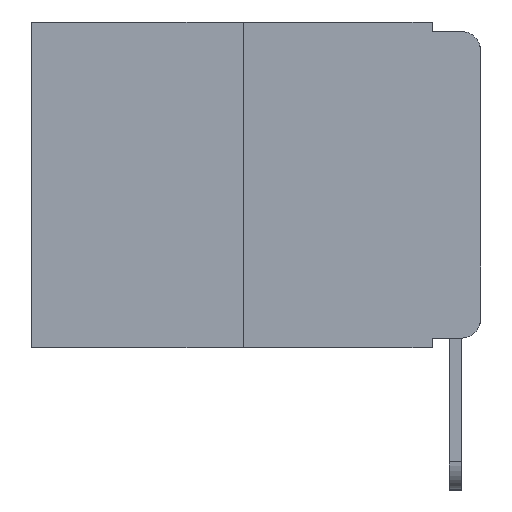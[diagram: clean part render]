
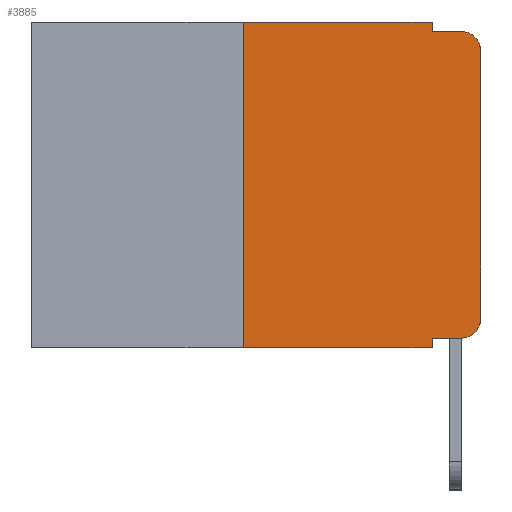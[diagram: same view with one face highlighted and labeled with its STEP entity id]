
A CAD part, left-side view. The second image highlights one B-rep face of the part: STEP entity #3885.
In plain terms, the highlighted planar face has unit normal (-1, 0, 0).
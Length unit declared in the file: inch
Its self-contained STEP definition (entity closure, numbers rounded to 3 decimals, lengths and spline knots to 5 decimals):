
#54 = DIRECTION ( 'NONE',  ( 0., 0., -1. ) ) ;
#356 = EDGE_CURVE ( 'NONE', #2292, #10760, #12862, .T. ) ;
#435 = VERTEX_POINT ( 'NONE', #4787 ) ;
#515 = VECTOR ( 'NONE', #8094, 39.37008 ) ;
#619 = EDGE_CURVE ( 'NONE', #8110, #1332, #3125, .T. ) ;
#902 = CARTESIAN_POINT ( 'NONE',  ( 0., 0.051, 0. ) ) ;
#1042 = ORIENTED_EDGE ( 'NONE', *, *, #1504, .T. ) ;
#1160 = VECTOR ( 'NONE', #5556, 39.37008 ) ;
#1332 = VERTEX_POINT ( 'NONE', #2573 ) ;
#1504 = EDGE_CURVE ( 'NONE', #435, #7835, #13304, .T. ) ;
#1597 = CARTESIAN_POINT ( 'NONE',  ( 0., 0.051, -0.333 ) ) ;
#1759 = EDGE_CURVE ( 'NONE', #7755, #8168, #12975, .T. ) ;
#1916 = PLANE ( 'NONE',  #10055 ) ;
#2100 = EDGE_CURVE ( 'NONE', #435, #2292, #2464, .T. ) ;
#2230 = CARTESIAN_POINT ( 'NONE',  ( 0., 0., -0.03 ) ) ;
#2292 = VERTEX_POINT ( 'NONE', #11133 ) ;
#2399 = CARTESIAN_POINT ( 'NONE',  ( 0., 0.051, -0.343 ) ) ;
#2464 = LINE ( 'NONE', #9834, #5792 ) ;
#2573 = CARTESIAN_POINT ( 'NONE',  ( 0., 0.02, -0.01 ) ) ;
#2598 = DIRECTION ( 'NONE',  ( 0., 0., 1. ) ) ;
#2879 = EDGE_CURVE ( 'NONE', #10760, #8481, #5236, .T. ) ;
#2931 = LINE ( 'NONE', #7078, #10517 ) ;
#3125 = CIRCLE ( 'NONE', #4054, 0.02 ) ;
#3409 = VECTOR ( 'NONE', #5769, 39.37008 ) ;
#3885 = ADVANCED_FACE ( 'NONE', ( #4985 ), #1916, .F. ) ;
#3945 = CARTESIAN_POINT ( 'NONE',  ( 0., 0.473, -0.343 ) ) ;
#4054 = AXIS2_PLACEMENT_3D ( 'NONE', #11546, #10380, #5473 ) ;
#4515 = CARTESIAN_POINT ( 'NONE',  ( 0., 0.051, -0.01 ) ) ;
#4525 = DIRECTION ( 'NONE',  ( 0., 0., -1. ) ) ;
#4658 = CARTESIAN_POINT ( 'NONE',  ( 0., 0.02, -0.313 ) ) ;
#4787 = CARTESIAN_POINT ( 'NONE',  ( 0., 0.25, -0.343 ) ) ;
#4985 = FACE_OUTER_BOUND ( 'NONE', #7806, .T. ) ;
#5236 = LINE ( 'NONE', #9388, #9660 ) ;
#5244 = ORIENTED_EDGE ( 'NONE', *, *, #8536, .T. ) ;
#5327 = DIRECTION ( 'NONE',  ( 0., -1., 0. ) ) ;
#5473 = DIRECTION ( 'NONE',  ( 0., 0., -1. ) ) ;
#5556 = DIRECTION ( 'NONE',  ( 0., -1., 0. ) ) ;
#5592 = EDGE_CURVE ( 'NONE', #6252, #7835, #2931, .T. ) ;
#5752 = CARTESIAN_POINT ( 'NONE',  ( 0., 0.473, 0. ) ) ;
#5769 = DIRECTION ( 'NONE',  ( 0., -1., 0. ) ) ;
#5792 = VECTOR ( 'NONE', #2598, 39.37008 ) ;
#6207 = CARTESIAN_POINT ( 'NONE',  ( 0., 0., 0. ) ) ;
#6252 = VERTEX_POINT ( 'NONE', #12806 ) ;
#6505 = VECTOR ( 'NONE', #9867, 39.37008 ) ;
#6750 = ORIENTED_EDGE ( 'NONE', *, *, #7826, .F. ) ;
#7059 = AXIS2_PLACEMENT_3D ( 'NONE', #4658, #13128, #4525 ) ;
#7078 = CARTESIAN_POINT ( 'NONE',  ( 0., 0.051, 0. ) ) ;
#7755 = VERTEX_POINT ( 'NONE', #12082 ) ;
#7806 = EDGE_LOOP ( 'NONE', ( #12119, #12657, #6750, #8155, #9506, #12696, #1042, #10019, #5244, #10357 ) ) ;
#7826 = EDGE_CURVE ( 'NONE', #8481, #1332, #8951, .T. ) ;
#7835 = VERTEX_POINT ( 'NONE', #2399 ) ;
#8094 = DIRECTION ( 'NONE',  ( 0., -1., 0. ) ) ;
#8110 = VERTEX_POINT ( 'NONE', #2230 ) ;
#8155 = ORIENTED_EDGE ( 'NONE', *, *, #2879, .F. ) ;
#8168 = VERTEX_POINT ( 'NONE', #12613 ) ;
#8182 = DIRECTION ( 'NONE',  ( 0., 0., -1. ) ) ;
#8481 = VERTEX_POINT ( 'NONE', #8971 ) ;
#8536 = EDGE_CURVE ( 'NONE', #6252, #7755, #11157, .T. ) ;
#8618 = VECTOR ( 'NONE', #5327, 39.37008 ) ;
#8951 = LINE ( 'NONE', #4515, #8618 ) ;
#8971 = CARTESIAN_POINT ( 'NONE',  ( 0., 0.051, -0.01 ) ) ;
#9388 = CARTESIAN_POINT ( 'NONE',  ( 0., 0.051, 0. ) ) ;
#9506 = ORIENTED_EDGE ( 'NONE', *, *, #356, .F. ) ;
#9660 = VECTOR ( 'NONE', #54, 39.37008 ) ;
#9834 = CARTESIAN_POINT ( 'NONE',  ( 0., 0.25, 0. ) ) ;
#9867 = DIRECTION ( 'NONE',  ( 0., 0., 1. ) ) ;
#10019 = ORIENTED_EDGE ( 'NONE', *, *, #5592, .F. ) ;
#10042 = CARTESIAN_POINT ( 'NONE',  ( 0., 0.473, 0. ) ) ;
#10055 = AXIS2_PLACEMENT_3D ( 'NONE', #10042, #10165, #8182 ) ;
#10165 = DIRECTION ( 'NONE',  ( 1., 0., 0. ) ) ;
#10357 = ORIENTED_EDGE ( 'NONE', *, *, #1759, .T. ) ;
#10380 = DIRECTION ( 'NONE',  ( -1., 0., 0. ) ) ;
#10517 = VECTOR ( 'NONE', #11332, 39.37008 ) ;
#10760 = VERTEX_POINT ( 'NONE', #902 ) ;
#11133 = CARTESIAN_POINT ( 'NONE',  ( 0., 0.25, 0. ) ) ;
#11157 = LINE ( 'NONE', #1597, #3409 ) ;
#11332 = DIRECTION ( 'NONE',  ( 0., 0., -1. ) ) ;
#11392 = LINE ( 'NONE', #6207, #6505 ) ;
#11546 = CARTESIAN_POINT ( 'NONE',  ( 0., 0.02, -0.03 ) ) ;
#12033 = EDGE_CURVE ( 'NONE', #8168, #8110, #11392, .T. ) ;
#12082 = CARTESIAN_POINT ( 'NONE',  ( 0., 0.02, -0.333 ) ) ;
#12119 = ORIENTED_EDGE ( 'NONE', *, *, #12033, .T. ) ;
#12613 = CARTESIAN_POINT ( 'NONE',  ( 0., 0., -0.313 ) ) ;
#12657 = ORIENTED_EDGE ( 'NONE', *, *, #619, .T. ) ;
#12696 = ORIENTED_EDGE ( 'NONE', *, *, #2100, .F. ) ;
#12806 = CARTESIAN_POINT ( 'NONE',  ( 0., 0.051, -0.333 ) ) ;
#12862 = LINE ( 'NONE', #5752, #1160 ) ;
#12975 = CIRCLE ( 'NONE', #7059, 0.02 ) ;
#13128 = DIRECTION ( 'NONE',  ( -1., 0., 0. ) ) ;
#13304 = LINE ( 'NONE', #3945, #515 ) ;
